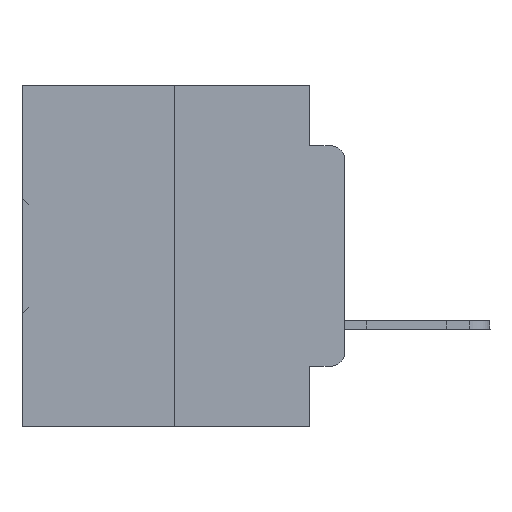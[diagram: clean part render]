
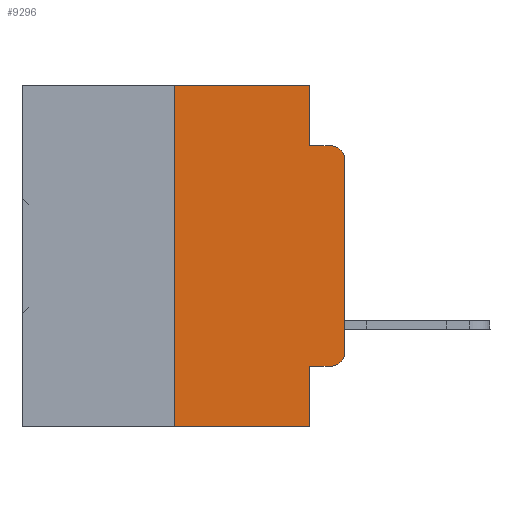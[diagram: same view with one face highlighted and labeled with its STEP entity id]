
A CAD part, left-side view. The second image highlights one B-rep face of the part: STEP entity #9296.
In plain terms, the highlighted planar face has unit normal (-1, 0, 0).
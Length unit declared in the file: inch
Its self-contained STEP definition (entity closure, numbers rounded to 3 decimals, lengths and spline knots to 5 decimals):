
#239 = CARTESIAN_POINT ( 'NONE',  ( 0., 0.051, -0.5 ) ) ;
#1682 = LINE ( 'NONE', #6165, #14029 ) ;
#1858 = DIRECTION ( 'NONE',  ( 0., 0., 1. ) ) ;
#1972 = DIRECTION ( 'NONE',  ( 0., 0., -1. ) ) ;
#2346 = EDGE_CURVE ( 'NONE', #8616, #37720, #14937, .T. ) ;
#2545 = DIRECTION ( 'NONE',  ( 1., 0., 0. ) ) ;
#2588 = EDGE_CURVE ( 'NONE', #3251, #3621, #1682, .T. ) ;
#3251 = VERTEX_POINT ( 'NONE', #37943 ) ;
#3621 = VERTEX_POINT ( 'NONE', #30338 ) ;
#3638 = VECTOR ( 'NONE', #23378, 39.37008 ) ;
#6102 = LINE ( 'NONE', #12749, #16139 ) ;
#6165 = CARTESIAN_POINT ( 'NONE',  ( 0., 0.25, 0. ) ) ;
#6296 = CARTESIAN_POINT ( 'NONE',  ( 0., 0.051, 0. ) ) ;
#6913 = ORIENTED_EDGE ( 'NONE', *, *, #2588, .F. ) ;
#7254 = CARTESIAN_POINT ( 'NONE',  ( 0., 0.02, -0.0885 ) ) ;
#7679 = DIRECTION ( 'NONE',  ( -1., 0., 0. ) ) ;
#7987 = PLANE ( 'NONE',  #24558 ) ;
#8139 = CARTESIAN_POINT ( 'NONE',  ( 0., 0., -0.3915 ) ) ;
#8171 = VECTOR ( 'NONE', #26818, 39.37008 ) ;
#8616 = VERTEX_POINT ( 'NONE', #10093 ) ;
#9188 = EDGE_LOOP ( 'NONE', ( #27368, #17333, #12261, #33103, #21342, #6913, #15528, #31275, #33125, #11071 ) ) ;
#9296 = ADVANCED_FACE ( 'NONE', ( #37652 ), #7987, .F. ) ;
#10093 = CARTESIAN_POINT ( 'NONE',  ( 0., 0.02, -0.4115 ) ) ;
#10510 = EDGE_CURVE ( 'NONE', #37720, #24066, #34857, .T. ) ;
#11071 = ORIENTED_EDGE ( 'NONE', *, *, #2346, .T. ) ;
#11896 = LINE ( 'NONE', #35589, #26591 ) ;
#12261 = ORIENTED_EDGE ( 'NONE', *, *, #35677, .F. ) ;
#12749 = CARTESIAN_POINT ( 'NONE',  ( 0., 0.473, -0.5 ) ) ;
#12955 = EDGE_CURVE ( 'NONE', #23901, #8616, #34136, .T. ) ;
#13332 = VERTEX_POINT ( 'NONE', #239 ) ;
#14029 = VECTOR ( 'NONE', #29386, 39.37008 ) ;
#14418 = CARTESIAN_POINT ( 'NONE',  ( 0., 0.02, -0.1085 ) ) ;
#14937 = CIRCLE ( 'NONE', #18654, 0.02 ) ;
#15528 = ORIENTED_EDGE ( 'NONE', *, *, #19521, .T. ) ;
#15826 = EDGE_CURVE ( 'NONE', #26126, #18745, #28861, .T. ) ;
#16139 = VECTOR ( 'NONE', #18259, 39.37008 ) ;
#16144 = CARTESIAN_POINT ( 'NONE',  ( 0., 0.051, -0.4115 ) ) ;
#16652 = CARTESIAN_POINT ( 'NONE',  ( 0., 0.02, -0.3915 ) ) ;
#17333 = ORIENTED_EDGE ( 'NONE', *, *, #24834, .T. ) ;
#17348 = DIRECTION ( 'NONE',  ( -1., 0., 0. ) ) ;
#17992 = AXIS2_PLACEMENT_3D ( 'NONE', #14418, #17348, #34584 ) ;
#18259 = DIRECTION ( 'NONE',  ( 0., -1., 0. ) ) ;
#18654 = AXIS2_PLACEMENT_3D ( 'NONE', #16652, #7679, #1972 ) ;
#18745 = VERTEX_POINT ( 'NONE', #20866 ) ;
#19521 = EDGE_CURVE ( 'NONE', #3251, #13332, #6102, .T. ) ;
#19581 = CARTESIAN_POINT ( 'NONE',  ( 0., 0.051, 0. ) ) ;
#20413 = CARTESIAN_POINT ( 'NONE',  ( 0., 0.051, 0. ) ) ;
#20866 = CARTESIAN_POINT ( 'NONE',  ( 0., 0.051, -0.0885 ) ) ;
#21342 = ORIENTED_EDGE ( 'NONE', *, *, #31526, .F. ) ;
#22011 = CARTESIAN_POINT ( 'NONE',  ( 0., 0.051, -0.0885 ) ) ;
#22201 = VECTOR ( 'NONE', #27150, 39.37008 ) ;
#23378 = DIRECTION ( 'NONE',  ( 0., 0., -1. ) ) ;
#23901 = VERTEX_POINT ( 'NONE', #16144 ) ;
#24066 = VERTEX_POINT ( 'NONE', #25514 ) ;
#24275 = LINE ( 'NONE', #20413, #3638 ) ;
#24558 = AXIS2_PLACEMENT_3D ( 'NONE', #28539, #2545, #34697 ) ;
#24834 = EDGE_CURVE ( 'NONE', #24066, #31213, #32218, .T. ) ;
#25514 = CARTESIAN_POINT ( 'NONE',  ( 0., 0., -0.1085 ) ) ;
#25605 = EDGE_CURVE ( 'NONE', #23901, #13332, #24275, .T. ) ;
#26126 = VERTEX_POINT ( 'NONE', #19581 ) ;
#26591 = VECTOR ( 'NONE', #26614, 39.37008 ) ;
#26614 = DIRECTION ( 'NONE',  ( 0., -1., 0. ) ) ;
#26818 = DIRECTION ( 'NONE',  ( 0., 0., -1. ) ) ;
#27150 = DIRECTION ( 'NONE',  ( 0., -1., 0. ) ) ;
#27368 = ORIENTED_EDGE ( 'NONE', *, *, #10510, .T. ) ;
#28539 = CARTESIAN_POINT ( 'NONE',  ( 0., 0.473, 0. ) ) ;
#28861 = LINE ( 'NONE', #6296, #8171 ) ;
#29386 = DIRECTION ( 'NONE',  ( 0., 0., 1. ) ) ;
#30338 = CARTESIAN_POINT ( 'NONE',  ( 0., 0.25, 0. ) ) ;
#30512 = DIRECTION ( 'NONE',  ( 0., -1., 0. ) ) ;
#31213 = VERTEX_POINT ( 'NONE', #7254 ) ;
#31275 = ORIENTED_EDGE ( 'NONE', *, *, #25605, .F. ) ;
#31526 = EDGE_CURVE ( 'NONE', #3621, #26126, #11896, .T. ) ;
#32218 = CIRCLE ( 'NONE', #17992, 0.02 ) ;
#32557 = LINE ( 'NONE', #22011, #36223 ) ;
#33103 = ORIENTED_EDGE ( 'NONE', *, *, #15826, .F. ) ;
#33125 = ORIENTED_EDGE ( 'NONE', *, *, #12955, .T. ) ;
#33433 = CARTESIAN_POINT ( 'NONE',  ( 0., 0.051, -0.4115 ) ) ;
#33638 = CARTESIAN_POINT ( 'NONE',  ( 0., 0., 0. ) ) ;
#33941 = VECTOR ( 'NONE', #1858, 39.37008 ) ;
#34136 = LINE ( 'NONE', #33433, #22201 ) ;
#34584 = DIRECTION ( 'NONE',  ( 0., 0., -1. ) ) ;
#34697 = DIRECTION ( 'NONE',  ( 0., 0., -1. ) ) ;
#34857 = LINE ( 'NONE', #33638, #33941 ) ;
#35589 = CARTESIAN_POINT ( 'NONE',  ( 0., 0.473, 0. ) ) ;
#35677 = EDGE_CURVE ( 'NONE', #18745, #31213, #32557, .T. ) ;
#36223 = VECTOR ( 'NONE', #30512, 39.37008 ) ;
#37652 = FACE_OUTER_BOUND ( 'NONE', #9188, .T. ) ;
#37720 = VERTEX_POINT ( 'NONE', #8139 ) ;
#37943 = CARTESIAN_POINT ( 'NONE',  ( 0., 0.25, -0.5 ) ) ;
